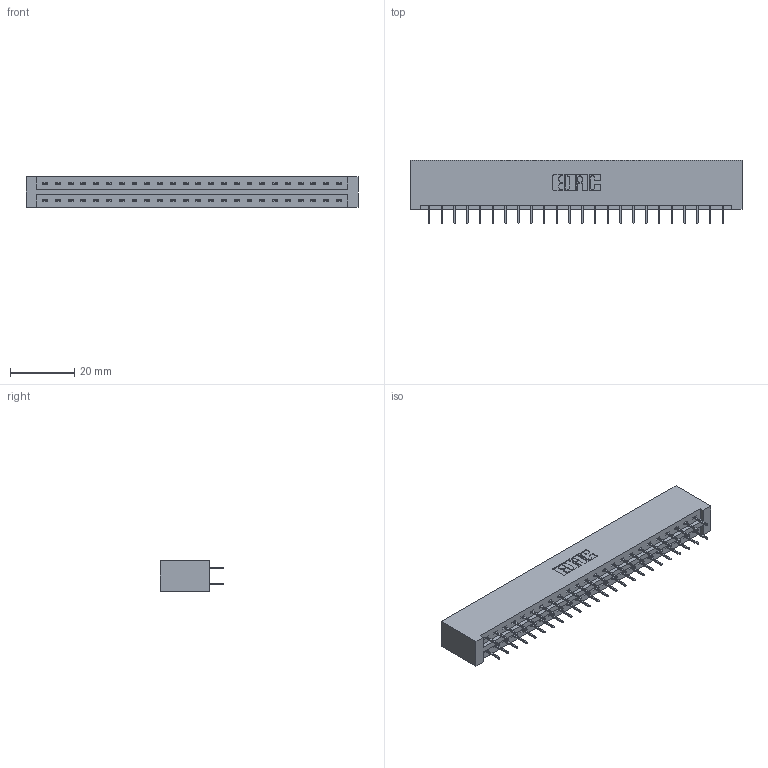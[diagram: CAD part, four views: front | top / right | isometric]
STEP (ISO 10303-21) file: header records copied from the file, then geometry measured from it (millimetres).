
FILE_DESCRIPTION (( 'STEP AP203' ), '1' );
FILE_NAME ('387-048-524-201.STEP', '2018-09-20T05:38:45', ( '' ), ( '' ), 'SwSTEP 2.0', 'SolidWorks 2016', '' );
FILE_SCHEMA (( 'CONFIG_CONTROL_DESIGN' ));
Length unit declared in the file: inch
Products named in the file (3): 337 Part_No Mounting Lugs; 345-292-001_345-293-124; 387-048-524-201
Assembly tree (49 placements, depth 2):
  387-048-524-201
    337 Part_No Mounting Lugs
    345-292-001_345-293-124  x48
Bounding box: 102.97 x 19.69 x 9.4 mm (x, y, z)
Volume: 11300.5 mm3; surface area: 12431.5 mm2
Topology: 49 solids, 49 shells, 2890 faces, 8207 edges, 5278 vertices
Faces by surface type: plane 2178, cylinder 712
Entity records: 20733 total; most frequent: CARTESIAN_POINT 3506, ORIENTED_EDGE 3442, DIRECTION 3009, EDGE_CURVE 1721, VECTOR 1605, LINE 1605, VERTEX_POINT 1142, AXIS2_PLACEMENT_3D 702
